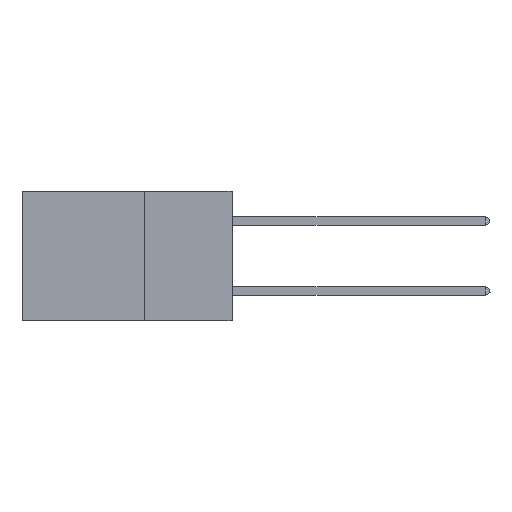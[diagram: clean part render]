
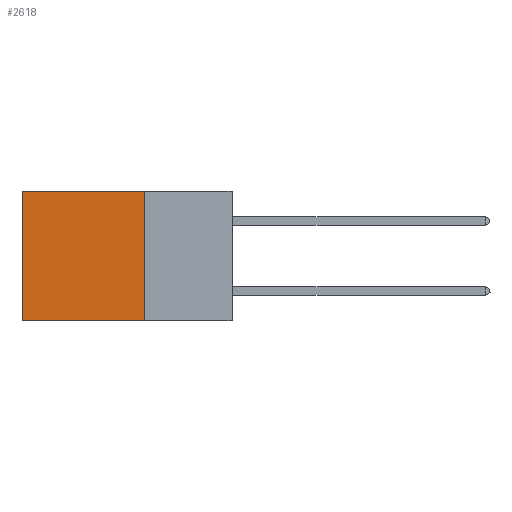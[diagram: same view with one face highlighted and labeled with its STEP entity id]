
A CAD part, left-side view. The second image highlights one B-rep face of the part: STEP entity #2618.
In plain terms, the highlighted planar face has unit normal (-1, 0, 0).
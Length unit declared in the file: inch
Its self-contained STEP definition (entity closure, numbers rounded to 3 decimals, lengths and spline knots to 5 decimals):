
#559 = AXIS2_PLACEMENT_3D ( 'NONE', #20583, #31014, #10315 ) ;
#1157 = ORIENTED_EDGE ( 'NONE', *, *, #29374, .F. ) ;
#2159 = CARTESIAN_POINT ( 'NONE',  ( 0.2875, 0.25, 0. ) ) ;
#2332 = VERTEX_POINT ( 'NONE', #36272 ) ;
#2460 = EDGE_CURVE ( 'NONE', #2332, #12993, #22507, .T. ) ;
#2618 = ADVANCED_FACE ( 'NONE', ( #16016 ), #6840, .F. ) ;
#3963 = VERTEX_POINT ( 'NONE', #28052 ) ;
#4991 = VECTOR ( 'NONE', #26364, 39.37008 ) ;
#5589 = CARTESIAN_POINT ( 'NONE',  ( 0.2875, 0.25, 0. ) ) ;
#5651 = VECTOR ( 'NONE', #21771, 39.37008 ) ;
#6840 = PLANE ( 'NONE',  #559 ) ;
#7598 = EDGE_CURVE ( 'NONE', #19003, #12993, #33225, .T. ) ;
#8821 = ORIENTED_EDGE ( 'NONE', *, *, #7598, .F. ) ;
#9652 = VECTOR ( 'NONE', #15888, 39.37008 ) ;
#10315 = DIRECTION ( 'NONE',  ( 0., 0., -1. ) ) ;
#12910 = DIRECTION ( 'NONE',  ( 0., 0., -1. ) ) ;
#12993 = VERTEX_POINT ( 'NONE', #17745 ) ;
#13127 = LINE ( 'NONE', #2159, #4991 ) ;
#14957 = EDGE_CURVE ( 'NONE', #3963, #2332, #13127, .T. ) ;
#15888 = DIRECTION ( 'NONE',  ( 0., 0., -1. ) ) ;
#16016 = FACE_OUTER_BOUND ( 'NONE', #26809, .T. ) ;
#17745 = CARTESIAN_POINT ( 'NONE',  ( 0.2875, 0.6, -0.37 ) ) ;
#18335 = CARTESIAN_POINT ( 'NONE',  ( 0.2875, 0.25, -0.37 ) ) ;
#19003 = VERTEX_POINT ( 'NONE', #28088 ) ;
#20583 = CARTESIAN_POINT ( 'NONE',  ( 0.2875, 0.25, 0. ) ) ;
#21771 = DIRECTION ( 'NONE',  ( 0., 1., 0. ) ) ;
#22507 = LINE ( 'NONE', #43800, #23588 ) ;
#23588 = VECTOR ( 'NONE', #12910, 39.37008 ) ;
#25892 = ORIENTED_EDGE ( 'NONE', *, *, #14957, .T. ) ;
#26364 = DIRECTION ( 'NONE',  ( 0., 1., 0. ) ) ;
#26809 = EDGE_LOOP ( 'NONE', ( #42429, #8821, #1157, #25892 ) ) ;
#28052 = CARTESIAN_POINT ( 'NONE',  ( 0.2875, 0.25, 0. ) ) ;
#28088 = CARTESIAN_POINT ( 'NONE',  ( 0.2875, 0.25, -0.37 ) ) ;
#29374 = EDGE_CURVE ( 'NONE', #3963, #19003, #36093, .T. ) ;
#31014 = DIRECTION ( 'NONE',  ( 1., 0., 0. ) ) ;
#33225 = LINE ( 'NONE', #18335, #5651 ) ;
#36093 = LINE ( 'NONE', #5589, #9652 ) ;
#36272 = CARTESIAN_POINT ( 'NONE',  ( 0.2875, 0.6, 0. ) ) ;
#42429 = ORIENTED_EDGE ( 'NONE', *, *, #2460, .T. ) ;
#43800 = CARTESIAN_POINT ( 'NONE',  ( 0.2875, 0.6, 0. ) ) ;
